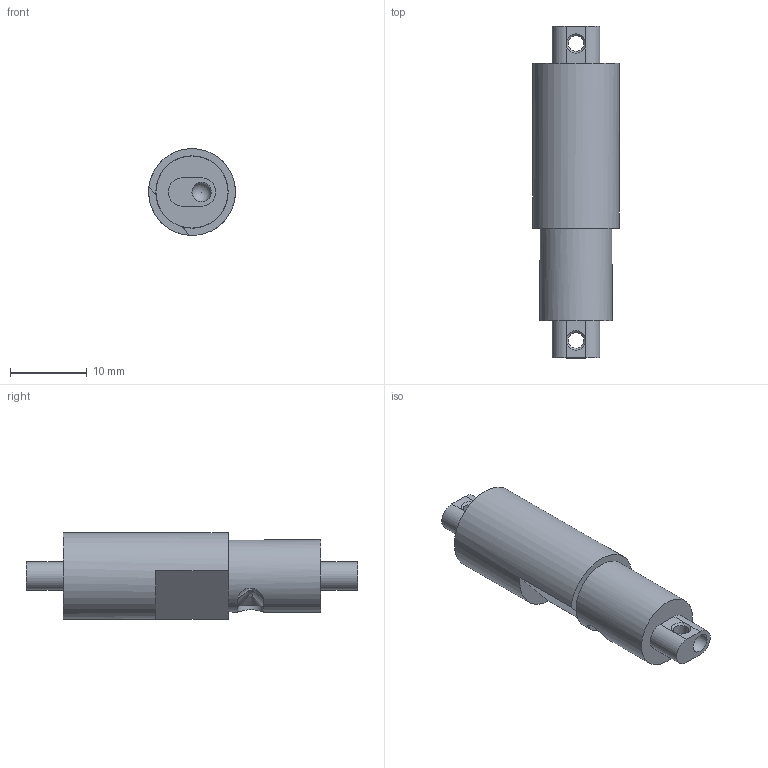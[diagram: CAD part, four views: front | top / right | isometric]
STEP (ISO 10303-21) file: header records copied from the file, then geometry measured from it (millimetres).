
FILE_DESCRIPTION(/* description */ (''),/* implementation_level */ '2;1');
FILE_NAME(/* name */ 'F Drum v19.step',/* time_stamp */ '2022-05-18T09:45:11-05:00',/* author */ (''),/* organization */ (''),/* preprocessor_version */ 'ST-DEVELOPER v18.1',/* originating_system */ 'Autodesk Translation Framework v10.14.0.1471',/* authorisation */ '');
FILE_SCHEMA (('AUTOMOTIVE_DESIGN { 1 0 10303 214 3 1 1 }'));
Length unit declared in the file: inch
Products named in the file (1): F Drum
Bounding box: 11.3 x 43.23 x 11.3 mm (x, y, z)
Volume: 3026.1 mm3; surface area: 1532.6 mm2
Topology: 1 solids, 1 shells, 39 faces, 117 edges, 76 vertices
Faces by surface type: plane 18, cylinder 11, cone 8, sphere 2
Full cylindrical faces by diameter (mm): 2.032 x2, 9.398 x1, 11.303 x1
Entity records: 1455 total; most frequent: CARTESIAN_POINT 385, ORIENTED_EDGE 226, DIRECTION 211, EDGE_CURVE 113, AXIS2_PLACEMENT_3D 83, VERTEX_POINT 76, LINE 45, VECTOR 45
